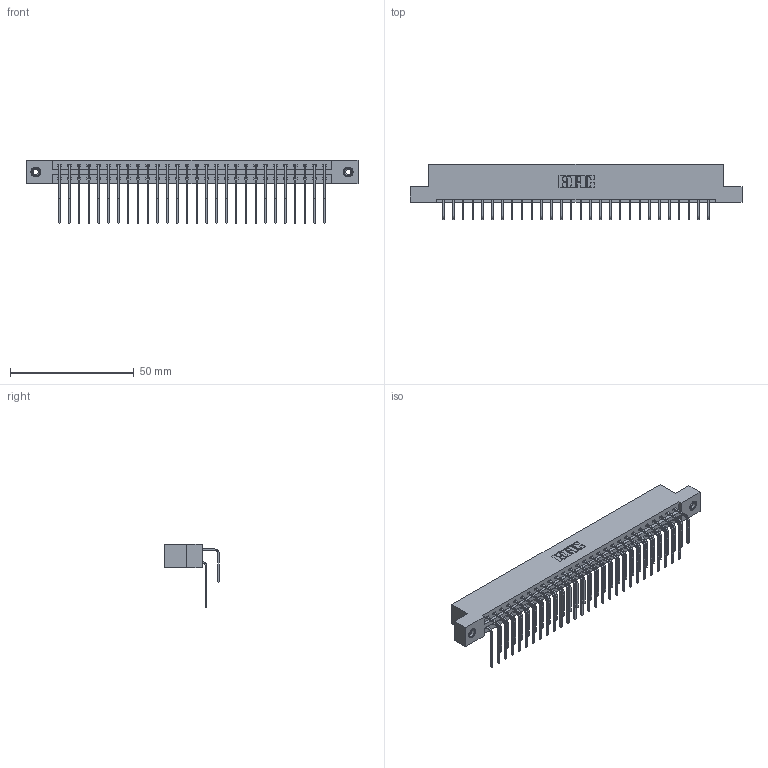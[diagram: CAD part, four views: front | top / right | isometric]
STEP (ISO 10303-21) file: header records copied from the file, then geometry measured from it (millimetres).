
FILE_DESCRIPTION (( 'STEP AP203' ), '1' );
FILE_NAME ('337-056-558-208.STEP', '2018-08-10T03:51:33', ( '' ), ( '' ), 'SwSTEP 2.0', 'SolidWorks 2016', '' );
FILE_SCHEMA (( 'CONFIG_CONTROL_DESIGN' ));
Length unit declared in the file: inch
Products named in the file (5): 345-250-001_345-250-003-102; 337-056-558-208; 337 Part_Flush Mounting Lugs - 0.156 Dia-TI; 345-292-001_558 559 Tail - 1; 345-292-001_558 Tail - 2
Assembly tree (59 placements, depth 2):
  337-056-558-208
    337 Part_Flush Mounting Lugs - 0.156 Dia-TI
    345-292-001_558 559 Tail - 1  x28
    345-292-001_558 Tail - 2  x28
    345-250-001_345-250-003-102  x2
Bounding box: 133.96 x 22.17 x 25.53 mm (x, y, z)
Volume: 14247.9 mm3; surface area: 17617.3 mm2
Topology: 59 solids, 59 shells, 3310 faces, 9799 edges, 6450 vertices
Faces by surface type: plane 2342, cylinder 952, cone 12, torus 4
Entity records: 26490 total; most frequent: CARTESIAN_POINT 4500, ORIENTED_EDGE 4378, DIRECTION 3867, EDGE_CURVE 2189, VECTOR 2001, LINE 2001, VERTEX_POINT 1452, AXIS2_PLACEMENT_3D 933
